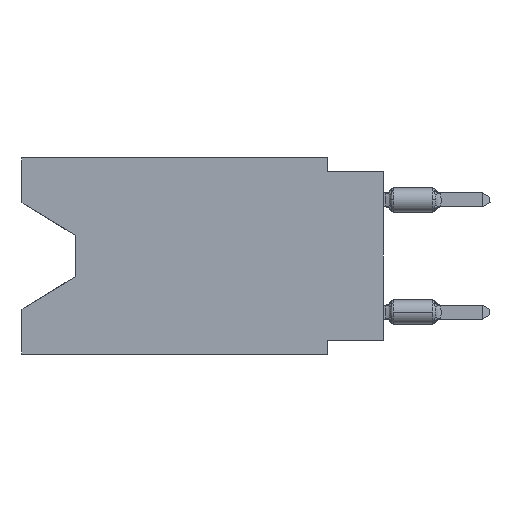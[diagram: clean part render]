
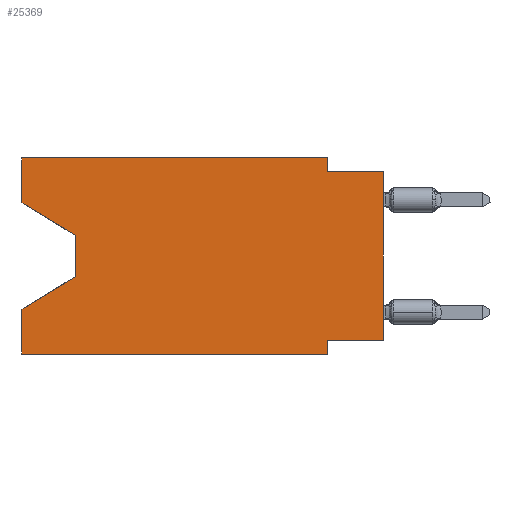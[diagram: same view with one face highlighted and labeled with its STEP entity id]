
A CAD part, left-side view. The second image highlights one B-rep face of the part: STEP entity #25369.
In plain terms, the highlighted planar face has unit normal (-1, 0, 0).
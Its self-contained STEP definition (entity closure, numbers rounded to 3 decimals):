
#264 = ORIENTED_EDGE ( 'NONE', *, *, #15159, .F. ) ;
#1087 = VECTOR ( 'NONE', #8218, 1000. ) ;
#1114 = VECTOR ( 'NONE', #15102, 1000. ) ;
#1254 = EDGE_LOOP ( 'NONE', ( #14853, #7470, #8983, #11179, #6373, #28524, #18514, #7953, #22687, #10948, #264, #15744 ) ) ;
#1418 = VECTOR ( 'NONE', #2081, 1000. ) ;
#1447 = CARTESIAN_POINT ( 'NONE',  ( 0., 16.383, -6.852 ) ) ;
#1522 = CARTESIAN_POINT ( 'NONE',  ( 0., 0., -8.255 ) ) ;
#1667 = LINE ( 'NONE', #1522, #1087 ) ;
#1714 = LINE ( 'NONE', #14826, #21967 ) ;
#1846 = EDGE_CURVE ( 'NONE', #11238, #16973, #5469, .T. ) ;
#2081 = DIRECTION ( 'NONE',  ( 0., 0.855, -0.519 ) ) ;
#3036 = VECTOR ( 'NONE', #17141, 1000. ) ;
#3052 = CARTESIAN_POINT ( 'NONE',  ( 0., 0., -8.255 ) ) ;
#3404 = DIRECTION ( 'NONE',  ( 0., -0.855, -0.519 ) ) ;
#3552 = VECTOR ( 'NONE', #3404, 1000. ) ;
#3792 = VERTEX_POINT ( 'NONE', #8517 ) ;
#4459 = CARTESIAN_POINT ( 'NONE',  ( 0., 16.383, -8.89 ) ) ;
#5150 = VECTOR ( 'NONE', #23644, 1000. ) ;
#5344 = VERTEX_POINT ( 'NONE', #10445 ) ;
#5469 = LINE ( 'NONE', #24077, #5150 ) ;
#5919 = DIRECTION ( 'NONE',  ( 0., 0., -1. ) ) ;
#6208 = LINE ( 'NONE', #12766, #14993 ) ;
#6373 = ORIENTED_EDGE ( 'NONE', *, *, #1846, .T. ) ;
#7168 = VERTEX_POINT ( 'NONE', #9525 ) ;
#7330 = VECTOR ( 'NONE', #12344, 1000. ) ;
#7470 = ORIENTED_EDGE ( 'NONE', *, *, #12779, .T. ) ;
#7769 = DIRECTION ( 'NONE',  ( 0., 0., -1. ) ) ;
#7953 = ORIENTED_EDGE ( 'NONE', *, *, #12421, .T. ) ;
#8020 = LINE ( 'NONE', #26208, #7330 ) ;
#8057 = LINE ( 'NONE', #12383, #3036 ) ;
#8218 = DIRECTION ( 'NONE',  ( 0., 1., 0. ) ) ;
#8517 = CARTESIAN_POINT ( 'NONE',  ( 0., 16.383, 0. ) ) ;
#8674 = CARTESIAN_POINT ( 'NONE',  ( 0., 16.383, 0. ) ) ;
#8837 = VERTEX_POINT ( 'NONE', #9946 ) ;
#8983 = ORIENTED_EDGE ( 'NONE', *, *, #24380, .T. ) ;
#9294 = VERTEX_POINT ( 'NONE', #3052 ) ;
#9525 = CARTESIAN_POINT ( 'NONE',  ( 0., 2.54, 0. ) ) ;
#9834 = EDGE_CURVE ( 'NONE', #9294, #22330, #1667, .T. ) ;
#9946 = CARTESIAN_POINT ( 'NONE',  ( 0., 13.97, -3.505 ) ) ;
#10281 = EDGE_CURVE ( 'NONE', #19377, #5344, #22108, .T. ) ;
#10383 = VECTOR ( 'NONE', #28858, 1000. ) ;
#10445 = CARTESIAN_POINT ( 'NONE',  ( 0., 0., -0.635 ) ) ;
#10497 = CARTESIAN_POINT ( 'NONE',  ( 0., 0., -0.635 ) ) ;
#10692 = CARTESIAN_POINT ( 'NONE',  ( 0., 16.383, 0. ) ) ;
#10948 = ORIENTED_EDGE ( 'NONE', *, *, #25575, .F. ) ;
#11179 = ORIENTED_EDGE ( 'NONE', *, *, #20516, .F. ) ;
#11238 = VERTEX_POINT ( 'NONE', #4459 ) ;
#12249 = PLANE ( 'NONE',  #25257 ) ;
#12344 = DIRECTION ( 'NONE',  ( 0., 0., -1. ) ) ;
#12383 = CARTESIAN_POINT ( 'NONE',  ( 0., 0., 0. ) ) ;
#12421 = EDGE_CURVE ( 'NONE', #9294, #5344, #8057, .T. ) ;
#12766 = CARTESIAN_POINT ( 'NONE',  ( 0., 2.54, -8.89 ) ) ;
#12779 = EDGE_CURVE ( 'NONE', #8837, #28086, #8020, .T. ) ;
#12782 = EDGE_CURVE ( 'NONE', #14488, #8837, #12794, .T. ) ;
#12794 = LINE ( 'NONE', #24111, #3552 ) ;
#14488 = VERTEX_POINT ( 'NONE', #24731 ) ;
#14826 = CARTESIAN_POINT ( 'NONE',  ( 0., 16.383, 0. ) ) ;
#14853 = ORIENTED_EDGE ( 'NONE', *, *, #12782, .T. ) ;
#14955 = LINE ( 'NONE', #8674, #25053 ) ;
#14993 = VECTOR ( 'NONE', #5919, 1000. ) ;
#15102 = DIRECTION ( 'NONE',  ( 0., -1., 0. ) ) ;
#15159 = EDGE_CURVE ( 'NONE', #3792, #7168, #14955, .T. ) ;
#15744 = ORIENTED_EDGE ( 'NONE', *, *, #26168, .F. ) ;
#16303 = CARTESIAN_POINT ( 'NONE',  ( 0., 2.54, -0.635 ) ) ;
#16973 = VERTEX_POINT ( 'NONE', #17877 ) ;
#17141 = DIRECTION ( 'NONE',  ( 0., 0., 1. ) ) ;
#17877 = CARTESIAN_POINT ( 'NONE',  ( 0., 2.54, -8.89 ) ) ;
#18514 = ORIENTED_EDGE ( 'NONE', *, *, #9834, .F. ) ;
#19084 = CARTESIAN_POINT ( 'NONE',  ( 0., 16.383, 0. ) ) ;
#19195 = CARTESIAN_POINT ( 'NONE',  ( 0., 13.97, -5.385 ) ) ;
#19377 = VERTEX_POINT ( 'NONE', #16303 ) ;
#19566 = DIRECTION ( 'NONE',  ( 0., -1., 0. ) ) ;
#19957 = LINE ( 'NONE', #24589, #24759 ) ;
#20516 = EDGE_CURVE ( 'NONE', #11238, #28562, #29429, .T. ) ;
#21967 = VECTOR ( 'NONE', #23920, 1000. ) ;
#22108 = LINE ( 'NONE', #10497, #1114 ) ;
#22330 = VERTEX_POINT ( 'NONE', #27767 ) ;
#22687 = ORIENTED_EDGE ( 'NONE', *, *, #10281, .F. ) ;
#23644 = DIRECTION ( 'NONE',  ( 0., -1., 0. ) ) ;
#23920 = DIRECTION ( 'NONE',  ( 0., 0., 1. ) ) ;
#24077 = CARTESIAN_POINT ( 'NONE',  ( 0., 16.383, -8.89 ) ) ;
#24111 = CARTESIAN_POINT ( 'NONE',  ( 0., 16.383, -2.038 ) ) ;
#24380 = EDGE_CURVE ( 'NONE', #28086, #28562, #26822, .T. ) ;
#24589 = CARTESIAN_POINT ( 'NONE',  ( 0., 2.54, 0. ) ) ;
#24731 = CARTESIAN_POINT ( 'NONE',  ( 0., 16.383, -2.038 ) ) ;
#24759 = VECTOR ( 'NONE', #27124, 1000. ) ;
#25053 = VECTOR ( 'NONE', #19566, 1000. ) ;
#25257 = AXIS2_PLACEMENT_3D ( 'NONE', #19084, #28181, #7769 ) ;
#25369 = ADVANCED_FACE ( 'NONE', ( #25808 ), #12249, .F. ) ;
#25575 = EDGE_CURVE ( 'NONE', #7168, #19377, #19957, .T. ) ;
#25808 = FACE_OUTER_BOUND ( 'NONE', #1254, .T. ) ;
#26168 = EDGE_CURVE ( 'NONE', #14488, #3792, #1714, .T. ) ;
#26208 = CARTESIAN_POINT ( 'NONE',  ( 0., 13.97, -3.505 ) ) ;
#26806 = EDGE_CURVE ( 'NONE', #22330, #16973, #6208, .T. ) ;
#26822 = LINE ( 'NONE', #27120, #1418 ) ;
#27120 = CARTESIAN_POINT ( 'NONE',  ( 0., 13.97, -5.385 ) ) ;
#27124 = DIRECTION ( 'NONE',  ( 0., 0., -1. ) ) ;
#27767 = CARTESIAN_POINT ( 'NONE',  ( 0., 2.54, -8.255 ) ) ;
#28086 = VERTEX_POINT ( 'NONE', #19195 ) ;
#28181 = DIRECTION ( 'NONE',  ( 1., 0., 0. ) ) ;
#28524 = ORIENTED_EDGE ( 'NONE', *, *, #26806, .F. ) ;
#28562 = VERTEX_POINT ( 'NONE', #1447 ) ;
#28858 = DIRECTION ( 'NONE',  ( 0., 0., 1. ) ) ;
#29429 = LINE ( 'NONE', #10692, #10383 ) ;
